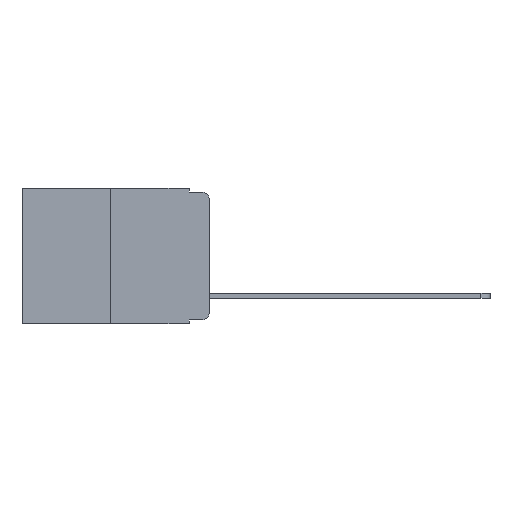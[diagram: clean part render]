
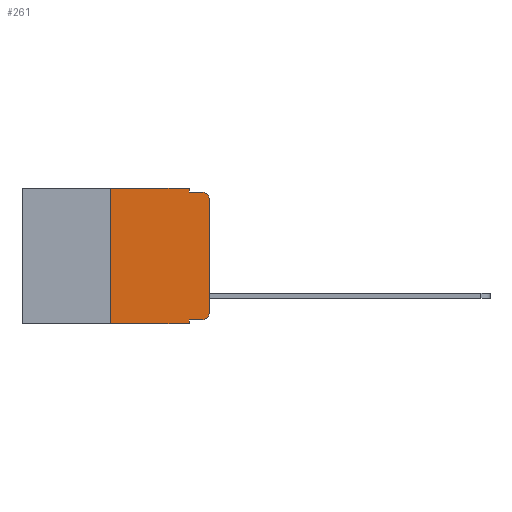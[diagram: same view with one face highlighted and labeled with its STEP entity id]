
A CAD part, left-side view. The second image highlights one B-rep face of the part: STEP entity #261.
In plain terms, the highlighted planar face has unit normal (-1, 0, 0).
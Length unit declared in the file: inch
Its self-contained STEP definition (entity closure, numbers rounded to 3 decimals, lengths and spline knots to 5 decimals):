
#56 = AXIS2_PLACEMENT_3D ( 'NONE', #724, #12774, #2502 ) ;
#112 = CARTESIAN_POINT ( 'NONE',  ( 0., 0.051, -0.333 ) ) ;
#261 = ADVANCED_FACE ( 'NONE', ( #4226 ), #6796, .F. ) ;
#655 = AXIS2_PLACEMENT_3D ( 'NONE', #6799, #20597, #18638 ) ;
#724 = CARTESIAN_POINT ( 'NONE',  ( 0., 0.02, -0.313 ) ) ;
#1144 = CARTESIAN_POINT ( 'NONE',  ( 0., 0.051, 0. ) ) ;
#1234 = AXIS2_PLACEMENT_3D ( 'NONE', #13244, #3007, #14896 ) ;
#1405 = CARTESIAN_POINT ( 'NONE',  ( 0., 0.25, -0.343 ) ) ;
#1483 = LINE ( 'NONE', #15028, #18883 ) ;
#1773 = DIRECTION ( 'NONE',  ( 0., 0., -1. ) ) ;
#1909 = DIRECTION ( 'NONE',  ( 0., -1., 0. ) ) ;
#2077 = DIRECTION ( 'NONE',  ( 0., 0., 1. ) ) ;
#2139 = VECTOR ( 'NONE', #2077, 39.37008 ) ;
#2502 = DIRECTION ( 'NONE',  ( 0., 0., -1. ) ) ;
#2689 = VERTEX_POINT ( 'NONE', #19108 ) ;
#3007 = DIRECTION ( 'NONE',  ( -1., 0., 0. ) ) ;
#3934 = LINE ( 'NONE', #21215, #7965 ) ;
#4226 = FACE_OUTER_BOUND ( 'NONE', #17904, .T. ) ;
#4874 = DIRECTION ( 'NONE',  ( 0., 0., 1. ) ) ;
#4887 = DIRECTION ( 'NONE',  ( 0., -1., 0. ) ) ;
#5812 = CARTESIAN_POINT ( 'NONE',  ( 0., 0.02, -0.01 ) ) ;
#5953 = CARTESIAN_POINT ( 'NONE',  ( 0., 0.051, -0.01 ) ) ;
#6424 = DIRECTION ( 'NONE',  ( 0., -1., 0. ) ) ;
#6796 = PLANE ( 'NONE',  #655 ) ;
#6799 = CARTESIAN_POINT ( 'NONE',  ( 0., 0.473, 0. ) ) ;
#7329 = CIRCLE ( 'NONE', #1234, 0.02 ) ;
#7455 = CARTESIAN_POINT ( 'NONE',  ( 0., 0.051, -0.01 ) ) ;
#7643 = LINE ( 'NONE', #5953, #11608 ) ;
#7775 = CARTESIAN_POINT ( 'NONE',  ( 0., 0.051, -0.343 ) ) ;
#7914 = LINE ( 'NONE', #9888, #20071 ) ;
#7965 = VECTOR ( 'NONE', #9657, 39.37008 ) ;
#8276 = VERTEX_POINT ( 'NONE', #1405 ) ;
#8380 = ORIENTED_EDGE ( 'NONE', *, *, #19494, .T. ) ;
#8771 = VECTOR ( 'NONE', #1773, 39.37008 ) ;
#8919 = ORIENTED_EDGE ( 'NONE', *, *, #17333, .F. ) ;
#9657 = DIRECTION ( 'NONE',  ( 0., 0., -1. ) ) ;
#9675 = VERTEX_POINT ( 'NONE', #18687 ) ;
#9888 = CARTESIAN_POINT ( 'NONE',  ( 0., 0.25, 0. ) ) ;
#10146 = LINE ( 'NONE', #17235, #18418 ) ;
#11009 = ORIENTED_EDGE ( 'NONE', *, *, #13254, .T. ) ;
#11123 = VERTEX_POINT ( 'NONE', #5812 ) ;
#11608 = VECTOR ( 'NONE', #19270, 39.37008 ) ;
#11816 = EDGE_CURVE ( 'NONE', #9675, #19170, #19444, .T. ) ;
#12077 = ORIENTED_EDGE ( 'NONE', *, *, #11816, .T. ) ;
#12235 = VECTOR ( 'NONE', #6424, 39.37008 ) ;
#12774 = DIRECTION ( 'NONE',  ( -1., 0., 0. ) ) ;
#12952 = EDGE_CURVE ( 'NONE', #19608, #9675, #10146, .T. ) ;
#13244 = CARTESIAN_POINT ( 'NONE',  ( 0., 0.02, -0.03 ) ) ;
#13254 = EDGE_CURVE ( 'NONE', #8276, #14345, #16633, .T. ) ;
#13931 = ORIENTED_EDGE ( 'NONE', *, *, #16810, .F. ) ;
#14059 = CARTESIAN_POINT ( 'NONE',  ( 0., 0., 0. ) ) ;
#14074 = EDGE_CURVE ( 'NONE', #19608, #14345, #17591, .T. ) ;
#14345 = VERTEX_POINT ( 'NONE', #7775 ) ;
#14654 = CARTESIAN_POINT ( 'NONE',  ( 0., 0.25, 0. ) ) ;
#14896 = DIRECTION ( 'NONE',  ( 0., 0., -1. ) ) ;
#15028 = CARTESIAN_POINT ( 'NONE',  ( 0., 0.473, 0. ) ) ;
#15168 = EDGE_CURVE ( 'NONE', #8276, #17272, #7914, .T. ) ;
#16458 = CARTESIAN_POINT ( 'NONE',  ( 0., 0.473, -0.343 ) ) ;
#16633 = LINE ( 'NONE', #16458, #12235 ) ;
#16741 = VERTEX_POINT ( 'NONE', #1144 ) ;
#16810 = EDGE_CURVE ( 'NONE', #17272, #16741, #1483, .T. ) ;
#17109 = VERTEX_POINT ( 'NONE', #7455 ) ;
#17235 = CARTESIAN_POINT ( 'NONE',  ( 0., 0.051, -0.333 ) ) ;
#17272 = VERTEX_POINT ( 'NONE', #14654 ) ;
#17333 = EDGE_CURVE ( 'NONE', #16741, #17109, #3934, .T. ) ;
#17591 = LINE ( 'NONE', #18307, #8771 ) ;
#17904 = EDGE_LOOP ( 'NONE', ( #20494, #8380, #21512, #8919, #13931, #18744, #11009, #19757, #20254, #12077 ) ) ;
#18307 = CARTESIAN_POINT ( 'NONE',  ( 0., 0.051, 0. ) ) ;
#18418 = VECTOR ( 'NONE', #1909, 39.37008 ) ;
#18421 = EDGE_CURVE ( 'NONE', #17109, #11123, #7643, .T. ) ;
#18638 = DIRECTION ( 'NONE',  ( 0., 0., -1. ) ) ;
#18687 = CARTESIAN_POINT ( 'NONE',  ( 0., 0.02, -0.333 ) ) ;
#18744 = ORIENTED_EDGE ( 'NONE', *, *, #15168, .F. ) ;
#18792 = CARTESIAN_POINT ( 'NONE',  ( 0., 0., -0.313 ) ) ;
#18883 = VECTOR ( 'NONE', #4887, 39.37008 ) ;
#19108 = CARTESIAN_POINT ( 'NONE',  ( 0., 0., -0.03 ) ) ;
#19170 = VERTEX_POINT ( 'NONE', #18792 ) ;
#19270 = DIRECTION ( 'NONE',  ( 0., -1., 0. ) ) ;
#19444 = CIRCLE ( 'NONE', #56, 0.02 ) ;
#19493 = LINE ( 'NONE', #14059, #2139 ) ;
#19494 = EDGE_CURVE ( 'NONE', #2689, #11123, #7329, .T. ) ;
#19608 = VERTEX_POINT ( 'NONE', #112 ) ;
#19757 = ORIENTED_EDGE ( 'NONE', *, *, #14074, .F. ) ;
#20071 = VECTOR ( 'NONE', #4874, 39.37008 ) ;
#20254 = ORIENTED_EDGE ( 'NONE', *, *, #12952, .T. ) ;
#20494 = ORIENTED_EDGE ( 'NONE', *, *, #20560, .T. ) ;
#20560 = EDGE_CURVE ( 'NONE', #19170, #2689, #19493, .T. ) ;
#20597 = DIRECTION ( 'NONE',  ( 1., 0., 0. ) ) ;
#21215 = CARTESIAN_POINT ( 'NONE',  ( 0., 0.051, 0. ) ) ;
#21512 = ORIENTED_EDGE ( 'NONE', *, *, #18421, .F. ) ;
